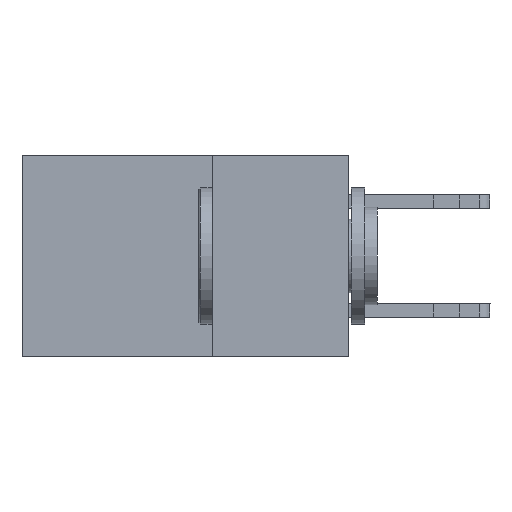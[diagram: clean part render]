
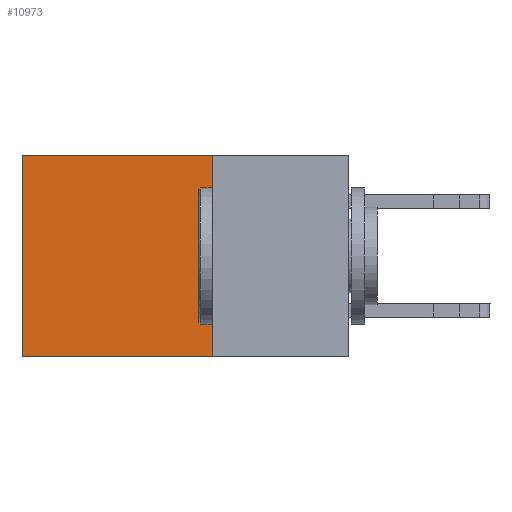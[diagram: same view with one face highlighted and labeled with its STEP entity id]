
A CAD part, left-side view. The second image highlights one B-rep face of the part: STEP entity #10973.
In plain terms, the highlighted planar face has unit normal (-1, 0, 0).
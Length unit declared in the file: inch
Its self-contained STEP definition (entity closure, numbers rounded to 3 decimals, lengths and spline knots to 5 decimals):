
#368 = LINE ( 'NONE', #9169, #918 ) ;
#483 = PLANE ( 'NONE',  #5318 ) ;
#918 = VECTOR ( 'NONE', #7434, 39.37008 ) ;
#965 = VECTOR ( 'NONE', #7806, 39.37008 ) ;
#1030 = CARTESIAN_POINT ( 'NONE',  ( 0.298, 0.25, 0. ) ) ;
#2235 = DIRECTION ( 'NONE',  ( 1., 0., 0. ) ) ;
#2637 = VECTOR ( 'NONE', #4492, 39.37008 ) ;
#2863 = CARTESIAN_POINT ( 'NONE',  ( 0.298, 0.6, 0. ) ) ;
#2991 = LINE ( 'NONE', #4568, #8189 ) ;
#3241 = CARTESIAN_POINT ( 'NONE',  ( 0.298, 0.25, 0. ) ) ;
#3345 = EDGE_LOOP ( 'NONE', ( #3455, #10651, #11360, #10178 ) ) ;
#3451 = VERTEX_POINT ( 'NONE', #4244 ) ;
#3455 = ORIENTED_EDGE ( 'NONE', *, *, #6585, .T. ) ;
#4006 = EDGE_CURVE ( 'NONE', #6881, #3451, #368, .T. ) ;
#4244 = CARTESIAN_POINT ( 'NONE',  ( 0.298, 0.6, -0.37 ) ) ;
#4492 = DIRECTION ( 'NONE',  ( 0., 0., -1. ) ) ;
#4568 = CARTESIAN_POINT ( 'NONE',  ( 0.298, 0.6, 0. ) ) ;
#5006 = VERTEX_POINT ( 'NONE', #1030 ) ;
#5067 = LINE ( 'NONE', #7888, #965 ) ;
#5318 = AXIS2_PLACEMENT_3D ( 'NONE', #3241, #2235, #5943 ) ;
#5943 = DIRECTION ( 'NONE',  ( 0., 0., -1. ) ) ;
#6585 = EDGE_CURVE ( 'NONE', #6694, #3451, #2991, .T. ) ;
#6694 = VERTEX_POINT ( 'NONE', #2863 ) ;
#6881 = VERTEX_POINT ( 'NONE', #10606 ) ;
#7263 = LINE ( 'NONE', #10086, #2637 ) ;
#7434 = DIRECTION ( 'NONE',  ( 0., 1., 0. ) ) ;
#7806 = DIRECTION ( 'NONE',  ( 0., 1., 0. ) ) ;
#7888 = CARTESIAN_POINT ( 'NONE',  ( 0.298, 0.25, 0. ) ) ;
#8189 = VECTOR ( 'NONE', #11011, 39.37008 ) ;
#9169 = CARTESIAN_POINT ( 'NONE',  ( 0.298, 0.25, -0.37 ) ) ;
#10086 = CARTESIAN_POINT ( 'NONE',  ( 0.298, 0.25, 0. ) ) ;
#10178 = ORIENTED_EDGE ( 'NONE', *, *, #11773, .T. ) ;
#10486 = FACE_OUTER_BOUND ( 'NONE', #3345, .T. ) ;
#10606 = CARTESIAN_POINT ( 'NONE',  ( 0.298, 0.25, -0.37 ) ) ;
#10651 = ORIENTED_EDGE ( 'NONE', *, *, #4006, .F. ) ;
#10742 = EDGE_CURVE ( 'NONE', #5006, #6881, #7263, .T. ) ;
#10973 = ADVANCED_FACE ( 'NONE', ( #10486 ), #483, .F. ) ;
#11011 = DIRECTION ( 'NONE',  ( 0., 0., -1. ) ) ;
#11360 = ORIENTED_EDGE ( 'NONE', *, *, #10742, .F. ) ;
#11773 = EDGE_CURVE ( 'NONE', #5006, #6694, #5067, .T. ) ;
